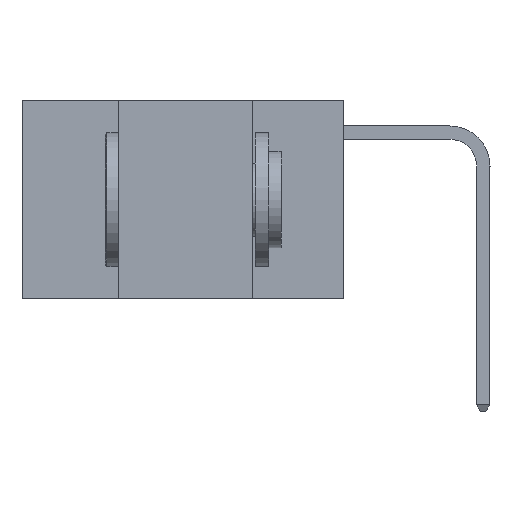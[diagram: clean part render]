
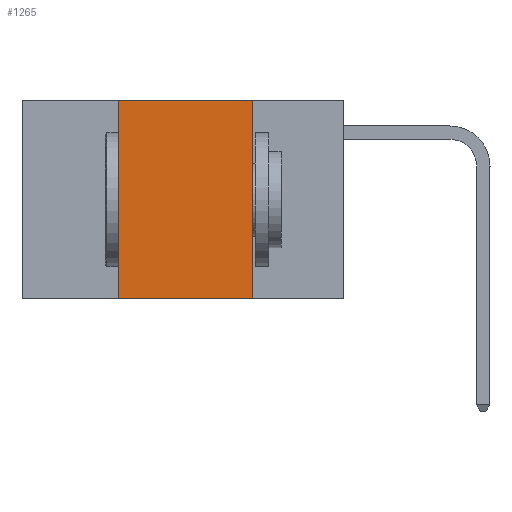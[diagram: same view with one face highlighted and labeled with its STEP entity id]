
A CAD part, left-side view. The second image highlights one B-rep face of the part: STEP entity #1265.
In plain terms, the highlighted planar face has unit normal (-1, 0, 0).
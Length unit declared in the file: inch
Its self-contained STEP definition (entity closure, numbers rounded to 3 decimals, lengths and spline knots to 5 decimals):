
#7 = CARTESIAN_POINT ( 'NONE',  ( 0., 0.6, -0.37 ) ) ;
#656 = LINE ( 'NONE', #7002, #10361 ) ;
#1265 = ADVANCED_FACE ( 'NONE', ( #10443 ), #1890, .F. ) ;
#1468 = ORIENTED_EDGE ( 'NONE', *, *, #3728, .F. ) ;
#1880 = VECTOR ( 'NONE', #7143, 39.37008 ) ;
#1890 = PLANE ( 'NONE',  #7572 ) ;
#2438 = LINE ( 'NONE', #7, #12101 ) ;
#2958 = DIRECTION ( 'NONE',  ( 0., 0., -1. ) ) ;
#3061 = CARTESIAN_POINT ( 'NONE',  ( 0., 0.17, 0. ) ) ;
#3085 = EDGE_LOOP ( 'NONE', ( #3972, #8986, #1468, #11608 ) ) ;
#3705 = EDGE_CURVE ( 'NONE', #4072, #5458, #656, .T. ) ;
#3728 = EDGE_CURVE ( 'NONE', #5995, #11587, #5748, .T. ) ;
#3746 = EDGE_CURVE ( 'NONE', #5995, #5458, #2438, .T. ) ;
#3972 = ORIENTED_EDGE ( 'NONE', *, *, #3705, .F. ) ;
#3993 = CARTESIAN_POINT ( 'NONE',  ( 0., 0.6, 0. ) ) ;
#4072 = VERTEX_POINT ( 'NONE', #3061 ) ;
#4143 = CARTESIAN_POINT ( 'NONE',  ( 0., 0.42, 0. ) ) ;
#4613 = CARTESIAN_POINT ( 'NONE',  ( 0., 0.42, 0. ) ) ;
#5068 = DIRECTION ( 'NONE',  ( 0., 0., -1. ) ) ;
#5458 = VERTEX_POINT ( 'NONE', #6109 ) ;
#5748 = LINE ( 'NONE', #4143, #8239 ) ;
#5995 = VERTEX_POINT ( 'NONE', #9672 ) ;
#6109 = CARTESIAN_POINT ( 'NONE',  ( 0., 0.17, -0.37 ) ) ;
#6174 = CARTESIAN_POINT ( 'NONE',  ( 0., 0.6, 0. ) ) ;
#7002 = CARTESIAN_POINT ( 'NONE',  ( 0., 0.17, 0. ) ) ;
#7092 = DIRECTION ( 'NONE',  ( 0., -1., 0. ) ) ;
#7143 = DIRECTION ( 'NONE',  ( 0., -1., 0. ) ) ;
#7572 = AXIS2_PLACEMENT_3D ( 'NONE', #3993, #8743, #2958 ) ;
#8239 = VECTOR ( 'NONE', #9732, 39.37008 ) ;
#8743 = DIRECTION ( 'NONE',  ( 1., 0., 0. ) ) ;
#8986 = ORIENTED_EDGE ( 'NONE', *, *, #11169, .F. ) ;
#9602 = LINE ( 'NONE', #6174, #1880 ) ;
#9672 = CARTESIAN_POINT ( 'NONE',  ( 0., 0.42, -0.37 ) ) ;
#9732 = DIRECTION ( 'NONE',  ( 0., 0., 1. ) ) ;
#10361 = VECTOR ( 'NONE', #5068, 39.37008 ) ;
#10443 = FACE_OUTER_BOUND ( 'NONE', #3085, .T. ) ;
#11169 = EDGE_CURVE ( 'NONE', #11587, #4072, #9602, .T. ) ;
#11587 = VERTEX_POINT ( 'NONE', #4613 ) ;
#11608 = ORIENTED_EDGE ( 'NONE', *, *, #3746, .T. ) ;
#12101 = VECTOR ( 'NONE', #7092, 39.37008 ) ;
